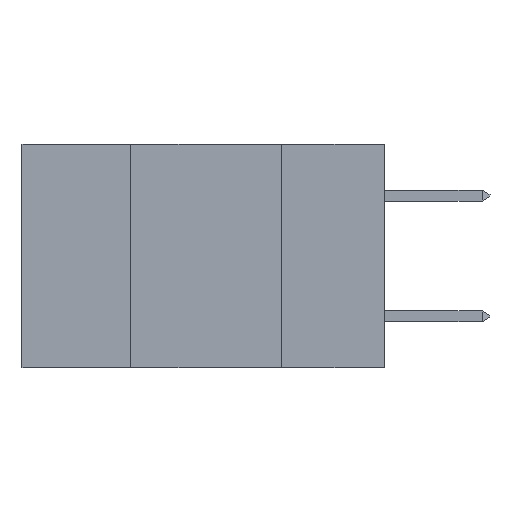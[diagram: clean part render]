
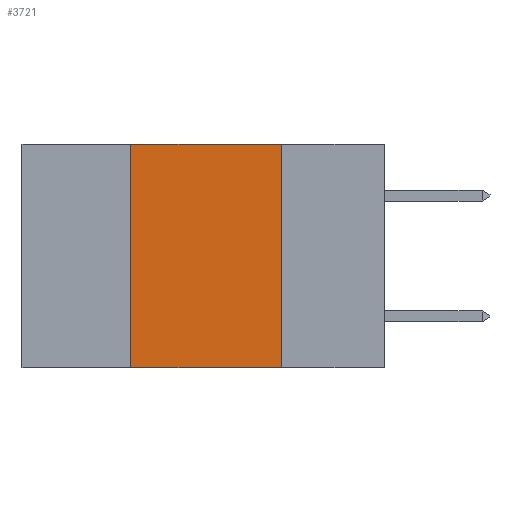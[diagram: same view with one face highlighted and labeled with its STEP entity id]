
A CAD part, left-side view. The second image highlights one B-rep face of the part: STEP entity #3721.
In plain terms, the highlighted planar face has unit normal (-1, 0, 0).
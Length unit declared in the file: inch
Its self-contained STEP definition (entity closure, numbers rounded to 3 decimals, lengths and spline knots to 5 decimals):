
#350 = CARTESIAN_POINT ( 'NONE',  ( 0., 0.17, 0. ) ) ;
#1026 = DIRECTION ( 'NONE',  ( 1., 0., 0. ) ) ;
#1034 = CARTESIAN_POINT ( 'NONE',  ( 0., 0.42, -0.37 ) ) ;
#1245 = ORIENTED_EDGE ( 'NONE', *, *, #7329, .F. ) ;
#1788 = DIRECTION ( 'NONE',  ( 0., 0., 1. ) ) ;
#1819 = CARTESIAN_POINT ( 'NONE',  ( 0., 0.17, 0. ) ) ;
#2622 = VECTOR ( 'NONE', #3536, 39.37008 ) ;
#2637 = VERTEX_POINT ( 'NONE', #1034 ) ;
#3536 = DIRECTION ( 'NONE',  ( 0., 0., -1. ) ) ;
#3615 = ORIENTED_EDGE ( 'NONE', *, *, #11468, .T. ) ;
#3721 = ADVANCED_FACE ( 'NONE', ( #4335 ), #4987, .F. ) ;
#4061 = VECTOR ( 'NONE', #1788, 39.37008 ) ;
#4335 = FACE_OUTER_BOUND ( 'NONE', #5718, .T. ) ;
#4791 = VERTEX_POINT ( 'NONE', #12589 ) ;
#4932 = EDGE_CURVE ( 'NONE', #9285, #10051, #9935, .T. ) ;
#4987 = PLANE ( 'NONE',  #8886 ) ;
#5661 = VECTOR ( 'NONE', #7434, 39.37008 ) ;
#5718 = EDGE_LOOP ( 'NONE', ( #11980, #1245, #7477, #3615 ) ) ;
#5959 = CARTESIAN_POINT ( 'NONE',  ( 0., 0.6, 0. ) ) ;
#6068 = LINE ( 'NONE', #11439, #8586 ) ;
#6354 = DIRECTION ( 'NONE',  ( 0., -1., 0. ) ) ;
#7329 = EDGE_CURVE ( 'NONE', #4791, #9285, #10523, .T. ) ;
#7434 = DIRECTION ( 'NONE',  ( 0., -1., 0. ) ) ;
#7456 = LINE ( 'NONE', #10739, #4061 ) ;
#7477 = ORIENTED_EDGE ( 'NONE', *, *, #11595, .F. ) ;
#8586 = VECTOR ( 'NONE', #6354, 39.37008 ) ;
#8886 = AXIS2_PLACEMENT_3D ( 'NONE', #5959, #1026, #8966 ) ;
#8966 = DIRECTION ( 'NONE',  ( 0., 0., -1. ) ) ;
#9285 = VERTEX_POINT ( 'NONE', #1819 ) ;
#9935 = LINE ( 'NONE', #350, #2622 ) ;
#10051 = VERTEX_POINT ( 'NONE', #11341 ) ;
#10523 = LINE ( 'NONE', #12482, #5661 ) ;
#10739 = CARTESIAN_POINT ( 'NONE',  ( 0., 0.42, 0. ) ) ;
#11341 = CARTESIAN_POINT ( 'NONE',  ( 0., 0.17, -0.37 ) ) ;
#11439 = CARTESIAN_POINT ( 'NONE',  ( 0., 0.6, -0.37 ) ) ;
#11468 = EDGE_CURVE ( 'NONE', #2637, #10051, #6068, .T. ) ;
#11595 = EDGE_CURVE ( 'NONE', #2637, #4791, #7456, .T. ) ;
#11980 = ORIENTED_EDGE ( 'NONE', *, *, #4932, .F. ) ;
#12482 = CARTESIAN_POINT ( 'NONE',  ( 0., 0.6, 0. ) ) ;
#12589 = CARTESIAN_POINT ( 'NONE',  ( 0., 0.42, 0. ) ) ;
